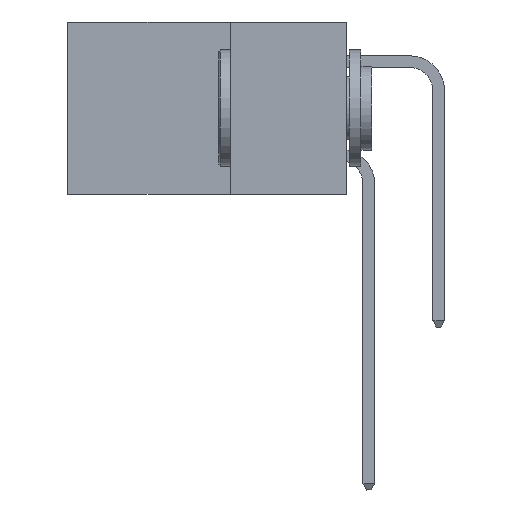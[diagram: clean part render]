
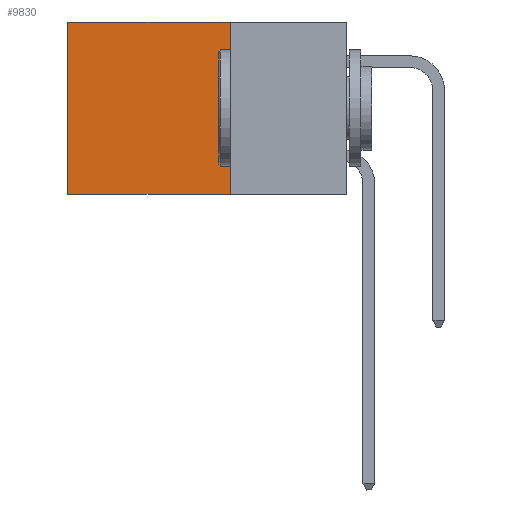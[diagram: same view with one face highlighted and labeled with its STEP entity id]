
A CAD part, left-side view. The second image highlights one B-rep face of the part: STEP entity #9830.
In plain terms, the highlighted planar face has unit normal (-1, 0, 0).
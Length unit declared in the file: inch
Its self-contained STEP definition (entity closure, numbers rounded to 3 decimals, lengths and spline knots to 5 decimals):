
#341 = DIRECTION ( 'NONE',  ( 0., 1., 0. ) ) ;
#667 = CARTESIAN_POINT ( 'NONE',  ( 0.2875, 0.6, 0. ) ) ;
#998 = DIRECTION ( 'NONE',  ( 0., 0., -1. ) ) ;
#2240 = DIRECTION ( 'NONE',  ( 0., 1., 0. ) ) ;
#2954 = LINE ( 'NONE', #11581, #13730 ) ;
#3691 = VECTOR ( 'NONE', #341, 39.37008 ) ;
#3728 = FACE_OUTER_BOUND ( 'NONE', #16129, .T. ) ;
#3964 = CARTESIAN_POINT ( 'NONE',  ( 0.2875, 0.25, 0. ) ) ;
#4137 = CARTESIAN_POINT ( 'NONE',  ( 0.2875, 0.6, 0. ) ) ;
#4433 = VECTOR ( 'NONE', #18029, 39.37008 ) ;
#4694 = VERTEX_POINT ( 'NONE', #12991 ) ;
#4989 = EDGE_CURVE ( 'NONE', #4694, #9947, #5936, .T. ) ;
#5787 = CARTESIAN_POINT ( 'NONE',  ( 0.2875, 0.25, -0.37 ) ) ;
#5936 = LINE ( 'NONE', #5787, #3691 ) ;
#8936 = EDGE_CURVE ( 'NONE', #15747, #4694, #2954, .T. ) ;
#9110 = LINE ( 'NONE', #4137, #4433 ) ;
#9830 = ADVANCED_FACE ( 'NONE', ( #3728 ), #15548, .F. ) ;
#9947 = VERTEX_POINT ( 'NONE', #10982 ) ;
#9952 = VECTOR ( 'NONE', #2240, 39.37008 ) ;
#10982 = CARTESIAN_POINT ( 'NONE',  ( 0.2875, 0.6, -0.37 ) ) ;
#11395 = AXIS2_PLACEMENT_3D ( 'NONE', #19068, #12026, #13806 ) ;
#11581 = CARTESIAN_POINT ( 'NONE',  ( 0.2875, 0.25, 0. ) ) ;
#12026 = DIRECTION ( 'NONE',  ( 1., 0., 0. ) ) ;
#12991 = CARTESIAN_POINT ( 'NONE',  ( 0.2875, 0.25, -0.37 ) ) ;
#13319 = ORIENTED_EDGE ( 'NONE', *, *, #8936, .F. ) ;
#13730 = VECTOR ( 'NONE', #998, 39.37008 ) ;
#13760 = ORIENTED_EDGE ( 'NONE', *, *, #15310, .T. ) ;
#13802 = VERTEX_POINT ( 'NONE', #667 ) ;
#13806 = DIRECTION ( 'NONE',  ( 0., 0., -1. ) ) ;
#13960 = ORIENTED_EDGE ( 'NONE', *, *, #15070, .T. ) ;
#13999 = CARTESIAN_POINT ( 'NONE',  ( 0.2875, 0.25, 0. ) ) ;
#14640 = LINE ( 'NONE', #3964, #9952 ) ;
#15070 = EDGE_CURVE ( 'NONE', #13802, #9947, #9110, .T. ) ;
#15310 = EDGE_CURVE ( 'NONE', #15747, #13802, #14640, .T. ) ;
#15548 = PLANE ( 'NONE',  #11395 ) ;
#15747 = VERTEX_POINT ( 'NONE', #13999 ) ;
#16129 = EDGE_LOOP ( 'NONE', ( #13960, #20264, #13319, #13760 ) ) ;
#18029 = DIRECTION ( 'NONE',  ( 0., 0., -1. ) ) ;
#19068 = CARTESIAN_POINT ( 'NONE',  ( 0.2875, 0.25, 0. ) ) ;
#20264 = ORIENTED_EDGE ( 'NONE', *, *, #4989, .F. ) ;
